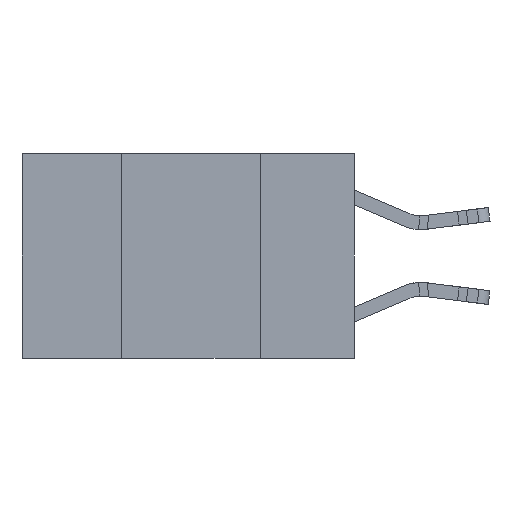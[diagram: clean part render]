
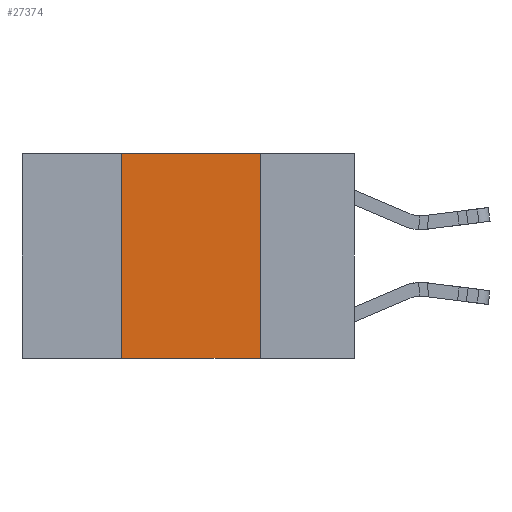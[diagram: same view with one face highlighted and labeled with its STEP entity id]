
A CAD part, left-side view. The second image highlights one B-rep face of the part: STEP entity #27374.
In plain terms, the highlighted planar face has unit normal (-1, 0, 0).
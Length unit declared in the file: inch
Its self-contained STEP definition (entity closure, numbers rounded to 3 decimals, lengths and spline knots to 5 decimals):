
#2113 = ORIENTED_EDGE ( 'NONE', *, *, #26615, .F. ) ;
#2186 = CARTESIAN_POINT ( 'NONE',  ( 0., 0.17, -0.37 ) ) ;
#2738 = LINE ( 'NONE', #8095, #10517 ) ;
#4905 = FACE_OUTER_BOUND ( 'NONE', #12977, .T. ) ;
#6331 = VECTOR ( 'NONE', #15687, 39.37008 ) ;
#7439 = LINE ( 'NONE', #17829, #20632 ) ;
#8095 = CARTESIAN_POINT ( 'NONE',  ( 0., 0.6, 0. ) ) ;
#9712 = VERTEX_POINT ( 'NONE', #2186 ) ;
#10511 = DIRECTION ( 'NONE',  ( 0., -1., 0. ) ) ;
#10517 = VECTOR ( 'NONE', #22174, 39.37008 ) ;
#10845 = PLANE ( 'NONE',  #18274 ) ;
#11124 = VERTEX_POINT ( 'NONE', #16619 ) ;
#12977 = EDGE_LOOP ( 'NONE', ( #22051, #2113, #20185, #23879 ) ) ;
#13168 = CARTESIAN_POINT ( 'NONE',  ( 0., 0.6, 0. ) ) ;
#13334 = CARTESIAN_POINT ( 'NONE',  ( 0., 0.17, 0. ) ) ;
#14810 = VERTEX_POINT ( 'NONE', #26730 ) ;
#15364 = EDGE_CURVE ( 'NONE', #14810, #15882, #7439, .T. ) ;
#15516 = DIRECTION ( 'NONE',  ( 0., 0., -1. ) ) ;
#15687 = DIRECTION ( 'NONE',  ( 0., 0., -1. ) ) ;
#15882 = VERTEX_POINT ( 'NONE', #19568 ) ;
#16619 = CARTESIAN_POINT ( 'NONE',  ( 0., 0.17, 0. ) ) ;
#17829 = CARTESIAN_POINT ( 'NONE',  ( 0., 0.42, 0. ) ) ;
#18274 = AXIS2_PLACEMENT_3D ( 'NONE', #13168, #29607, #15516 ) ;
#19568 = CARTESIAN_POINT ( 'NONE',  ( 0., 0.42, 0. ) ) ;
#20185 = ORIENTED_EDGE ( 'NONE', *, *, #15364, .F. ) ;
#20190 = DIRECTION ( 'NONE',  ( 0., 0., 1. ) ) ;
#20632 = VECTOR ( 'NONE', #20190, 39.37008 ) ;
#21791 = VECTOR ( 'NONE', #10511, 39.37008 ) ;
#22051 = ORIENTED_EDGE ( 'NONE', *, *, #22583, .F. ) ;
#22174 = DIRECTION ( 'NONE',  ( 0., -1., 0. ) ) ;
#22467 = EDGE_CURVE ( 'NONE', #14810, #9712, #28016, .T. ) ;
#22583 = EDGE_CURVE ( 'NONE', #11124, #9712, #25086, .T. ) ;
#23879 = ORIENTED_EDGE ( 'NONE', *, *, #22467, .T. ) ;
#24680 = CARTESIAN_POINT ( 'NONE',  ( 0., 0.6, -0.37 ) ) ;
#25086 = LINE ( 'NONE', #13334, #6331 ) ;
#26615 = EDGE_CURVE ( 'NONE', #15882, #11124, #2738, .T. ) ;
#26730 = CARTESIAN_POINT ( 'NONE',  ( 0., 0.42, -0.37 ) ) ;
#27374 = ADVANCED_FACE ( 'NONE', ( #4905 ), #10845, .F. ) ;
#28016 = LINE ( 'NONE', #24680, #21791 ) ;
#29607 = DIRECTION ( 'NONE',  ( 1., 0., 0. ) ) ;
